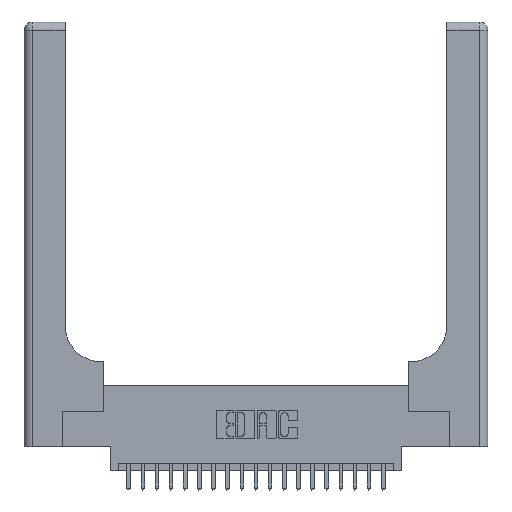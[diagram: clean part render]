
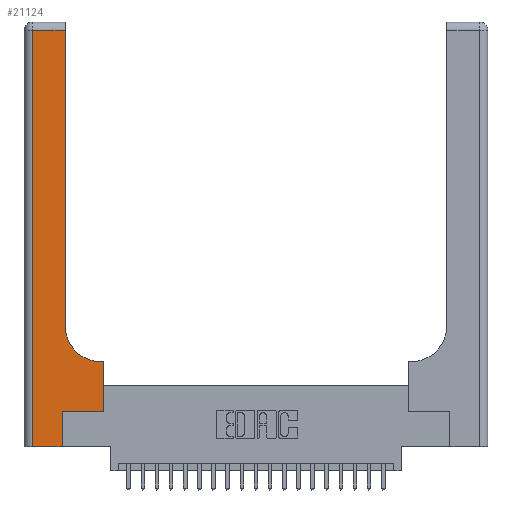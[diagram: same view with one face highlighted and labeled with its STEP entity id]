
A CAD part, top view. The second image highlights one B-rep face of the part: STEP entity #21124.
In plain terms, the highlighted planar face has unit normal (0, 0, 1).
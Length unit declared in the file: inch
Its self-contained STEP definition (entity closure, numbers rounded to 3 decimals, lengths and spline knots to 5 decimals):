
#659 = EDGE_CURVE ( 'NONE', #6284, #18027, #6242, .T. ) ;
#863 = CARTESIAN_POINT ( 'NONE',  ( 0.269, 0., 0.37 ) ) ;
#1246 = VERTEX_POINT ( 'NONE', #14215 ) ;
#1250 = VECTOR ( 'NONE', #6226, 39.37008 ) ;
#1896 = CARTESIAN_POINT ( 'NONE',  ( 0.2915, 0.6, 0.37 ) ) ;
#2042 = CARTESIAN_POINT ( 'NONE',  ( 0., 0., 0.37 ) ) ;
#2562 = EDGE_CURVE ( 'NONE', #3885, #21277, #4109, .T. ) ;
#3334 = EDGE_CURVE ( 'NONE', #4733, #7984, #16350, .T. ) ;
#3733 = ORIENTED_EDGE ( 'NONE', *, *, #19953, .T. ) ;
#3773 = CARTESIAN_POINT ( 'NONE',  ( 0.269, 0., 0.37 ) ) ;
#3885 = VERTEX_POINT ( 'NONE', #12692 ) ;
#3912 = DIRECTION ( 'NONE',  ( 0., 0., -1. ) ) ;
#4109 = LINE ( 'NONE', #12666, #12749 ) ;
#4344 = CARTESIAN_POINT ( 'NONE',  ( 0.06, 3., 0.37 ) ) ;
#4733 = VERTEX_POINT ( 'NONE', #10066 ) ;
#5011 = DIRECTION ( 'NONE',  ( 0., 0., -1. ) ) ;
#5067 = VECTOR ( 'NONE', #13788, 39.37008 ) ;
#5640 = LINE ( 'NONE', #4344, #1250 ) ;
#6107 = FACE_OUTER_BOUND ( 'NONE', #20130, .T. ) ;
#6226 = DIRECTION ( 'NONE',  ( 0., -1., 0. ) ) ;
#6242 = LINE ( 'NONE', #7691, #15332 ) ;
#6284 = VERTEX_POINT ( 'NONE', #11223 ) ;
#7066 = ORIENTED_EDGE ( 'NONE', *, *, #14589, .T. ) ;
#7381 = VERTEX_POINT ( 'NONE', #15001 ) ;
#7691 = CARTESIAN_POINT ( 'NONE',  ( 0.2915, 3., 0.37 ) ) ;
#7739 = DIRECTION ( 'NONE',  ( 0., 1., 0. ) ) ;
#7984 = VERTEX_POINT ( 'NONE', #3773 ) ;
#8319 = ORIENTED_EDGE ( 'NONE', *, *, #659, .T. ) ;
#8623 = LINE ( 'NONE', #1896, #9775 ) ;
#8870 = CARTESIAN_POINT ( 'NONE',  ( 0.5585, 0.6, 0.37 ) ) ;
#9283 = VECTOR ( 'NONE', #13562, 39.37008 ) ;
#9583 = ORIENTED_EDGE ( 'NONE', *, *, #12352, .T. ) ;
#9775 = VECTOR ( 'NONE', #14770, 39.37008 ) ;
#9975 = EDGE_CURVE ( 'NONE', #1246, #4733, #5640, .T. ) ;
#10066 = CARTESIAN_POINT ( 'NONE',  ( 0.06, 0., 0.37 ) ) ;
#10540 = PLANE ( 'NONE',  #19503 ) ;
#10555 = CARTESIAN_POINT ( 'NONE',  ( 0.2915, 2.94, 0.37 ) ) ;
#11223 = CARTESIAN_POINT ( 'NONE',  ( 0.2915, 0.85, 0.37 ) ) ;
#11324 = DIRECTION ( 'NONE',  ( 1., 0., 0. ) ) ;
#11484 = ORIENTED_EDGE ( 'NONE', *, *, #9975, .T. ) ;
#12352 = EDGE_CURVE ( 'NONE', #18027, #1246, #18769, .T. ) ;
#12653 = EDGE_CURVE ( 'NONE', #21277, #17526, #23076, .T. ) ;
#12666 = CARTESIAN_POINT ( 'NONE',  ( 0.269, 0.25, 0.37 ) ) ;
#12692 = CARTESIAN_POINT ( 'NONE',  ( 0.269, 0.25, 0.37 ) ) ;
#12749 = VECTOR ( 'NONE', #21354, 39.37008 ) ;
#13376 = ORIENTED_EDGE ( 'NONE', *, *, #17740, .T. ) ;
#13562 = DIRECTION ( 'NONE',  ( -1., 0., 0. ) ) ;
#13788 = DIRECTION ( 'NONE',  ( 0., 1., 0. ) ) ;
#14215 = CARTESIAN_POINT ( 'NONE',  ( 0.06, 2.94, 0.37 ) ) ;
#14589 = EDGE_CURVE ( 'NONE', #7984, #3885, #18335, .T. ) ;
#14770 = DIRECTION ( 'NONE',  ( -1., 0., 0. ) ) ;
#14872 = CARTESIAN_POINT ( 'NONE',  ( 0.5415, 0.85, 0.37 ) ) ;
#15001 = CARTESIAN_POINT ( 'NONE',  ( 0.5415, 0.6, 0.37 ) ) ;
#15332 = VECTOR ( 'NONE', #7739, 39.37008 ) ;
#15640 = CARTESIAN_POINT ( 'NONE',  ( 0.5585, 0.25, 0.37 ) ) ;
#15919 = CARTESIAN_POINT ( 'NONE',  ( 0., 3., 0.37 ) ) ;
#16350 = LINE ( 'NONE', #2042, #20940 ) ;
#16360 = ORIENTED_EDGE ( 'NONE', *, *, #3334, .T. ) ;
#16643 = DIRECTION ( 'NONE',  ( 1., 0., 0. ) ) ;
#17387 = VECTOR ( 'NONE', #17390, 39.37008 ) ;
#17390 = DIRECTION ( 'NONE',  ( 0., 1., 0. ) ) ;
#17526 = VERTEX_POINT ( 'NONE', #8870 ) ;
#17654 = DIRECTION ( 'NONE',  ( -1., 0., 0. ) ) ;
#17740 = EDGE_CURVE ( 'NONE', #7381, #6284, #21424, .T. ) ;
#18027 = VERTEX_POINT ( 'NONE', #10555 ) ;
#18335 = LINE ( 'NONE', #863, #5067 ) ;
#18766 = CARTESIAN_POINT ( 'NONE',  ( 0., 2.94, 0.37 ) ) ;
#18769 = LINE ( 'NONE', #18766, #9283 ) ;
#18972 = AXIS2_PLACEMENT_3D ( 'NONE', #14872, #3912, #16643 ) ;
#19503 = AXIS2_PLACEMENT_3D ( 'NONE', #15919, #5011, #17654 ) ;
#19842 = CARTESIAN_POINT ( 'NONE',  ( 0.5585, 0.25, 0.37 ) ) ;
#19953 = EDGE_CURVE ( 'NONE', #17526, #7381, #8623, .T. ) ;
#19966 = ORIENTED_EDGE ( 'NONE', *, *, #12653, .T. ) ;
#20130 = EDGE_LOOP ( 'NONE', ( #8319, #9583, #11484, #16360, #7066, #23354, #19966, #3733, #13376 ) ) ;
#20940 = VECTOR ( 'NONE', #11324, 39.37008 ) ;
#21124 = ADVANCED_FACE ( 'NONE', ( #6107 ), #10540, .F. ) ;
#21277 = VERTEX_POINT ( 'NONE', #19842 ) ;
#21354 = DIRECTION ( 'NONE',  ( 1., 0., 0. ) ) ;
#21424 = CIRCLE ( 'NONE', #18972, 0.25 ) ;
#23076 = LINE ( 'NONE', #15640, #17387 ) ;
#23354 = ORIENTED_EDGE ( 'NONE', *, *, #2562, .T. ) ;
